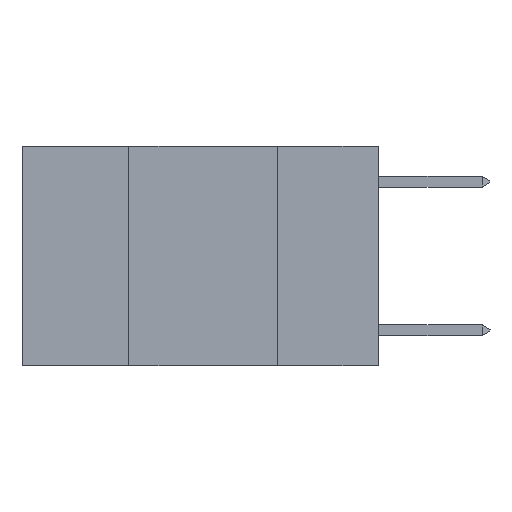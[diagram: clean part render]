
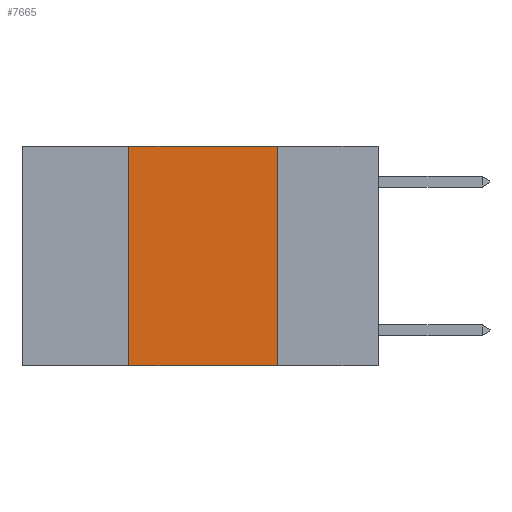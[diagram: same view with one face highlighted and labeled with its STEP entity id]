
A CAD part, left-side view. The second image highlights one B-rep face of the part: STEP entity #7665.
In plain terms, the highlighted planar face has unit normal (-1, 0, 0).
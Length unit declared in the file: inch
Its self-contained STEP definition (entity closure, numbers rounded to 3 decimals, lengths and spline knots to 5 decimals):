
#546 = VECTOR ( 'NONE', #2725, 39.37008 ) ;
#572 = CARTESIAN_POINT ( 'NONE',  ( 0., 0.6, 0. ) ) ;
#748 = DIRECTION ( 'NONE',  ( 0., 0., -1. ) ) ;
#798 = VERTEX_POINT ( 'NONE', #2781 ) ;
#1328 = DIRECTION ( 'NONE',  ( 0., 0., 1. ) ) ;
#1622 = DIRECTION ( 'NONE',  ( 1., 0., 0. ) ) ;
#2488 = AXIS2_PLACEMENT_3D ( 'NONE', #572, #1622, #8257 ) ;
#2567 = VECTOR ( 'NONE', #1328, 39.37008 ) ;
#2725 = DIRECTION ( 'NONE',  ( 0., -1., 0. ) ) ;
#2781 = CARTESIAN_POINT ( 'NONE',  ( 0., 0.42, -0.37 ) ) ;
#2809 = CARTESIAN_POINT ( 'NONE',  ( 0., 0.17, 0. ) ) ;
#2892 = LINE ( 'NONE', #2809, #4831 ) ;
#3167 = ORIENTED_EDGE ( 'NONE', *, *, #10740, .F. ) ;
#3221 = LINE ( 'NONE', #6454, #546 ) ;
#3280 = ORIENTED_EDGE ( 'NONE', *, *, #9564, .F. ) ;
#3355 = CARTESIAN_POINT ( 'NONE',  ( 0., 0.42, 0. ) ) ;
#3690 = EDGE_LOOP ( 'NONE', ( #3280, #4550, #3167, #6455 ) ) ;
#3724 = CARTESIAN_POINT ( 'NONE',  ( 0., 0.6, 0. ) ) ;
#3759 = CARTESIAN_POINT ( 'NONE',  ( 0., 0.42, 0. ) ) ;
#4550 = ORIENTED_EDGE ( 'NONE', *, *, #11926, .F. ) ;
#4831 = VECTOR ( 'NONE', #748, 39.37008 ) ;
#5023 = EDGE_CURVE ( 'NONE', #798, #7128, #3221, .T. ) ;
#6382 = PLANE ( 'NONE',  #2488 ) ;
#6401 = VERTEX_POINT ( 'NONE', #3759 ) ;
#6454 = CARTESIAN_POINT ( 'NONE',  ( 0., 0.6, -0.37 ) ) ;
#6455 = ORIENTED_EDGE ( 'NONE', *, *, #5023, .T. ) ;
#7128 = VERTEX_POINT ( 'NONE', #12001 ) ;
#7538 = LINE ( 'NONE', #3724, #9681 ) ;
#7665 = ADVANCED_FACE ( 'NONE', ( #10574 ), #6382, .F. ) ;
#8257 = DIRECTION ( 'NONE',  ( 0., 0., -1. ) ) ;
#9564 = EDGE_CURVE ( 'NONE', #11592, #7128, #2892, .T. ) ;
#9681 = VECTOR ( 'NONE', #11058, 39.37008 ) ;
#9703 = LINE ( 'NONE', #3355, #2567 ) ;
#10574 = FACE_OUTER_BOUND ( 'NONE', #3690, .T. ) ;
#10678 = CARTESIAN_POINT ( 'NONE',  ( 0., 0.17, 0. ) ) ;
#10740 = EDGE_CURVE ( 'NONE', #798, #6401, #9703, .T. ) ;
#11058 = DIRECTION ( 'NONE',  ( 0., -1., 0. ) ) ;
#11592 = VERTEX_POINT ( 'NONE', #10678 ) ;
#11926 = EDGE_CURVE ( 'NONE', #6401, #11592, #7538, .T. ) ;
#12001 = CARTESIAN_POINT ( 'NONE',  ( 0., 0.17, -0.37 ) ) ;
